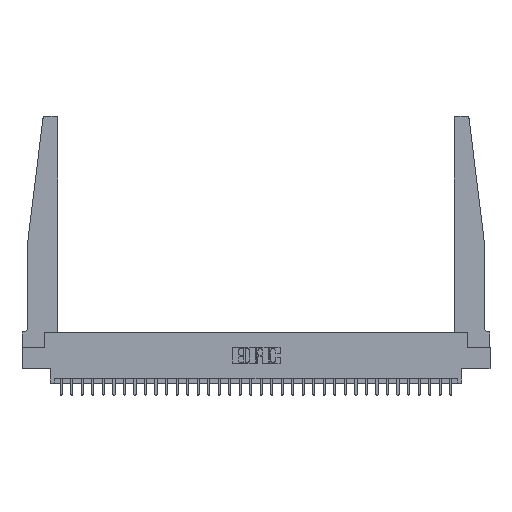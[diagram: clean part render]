
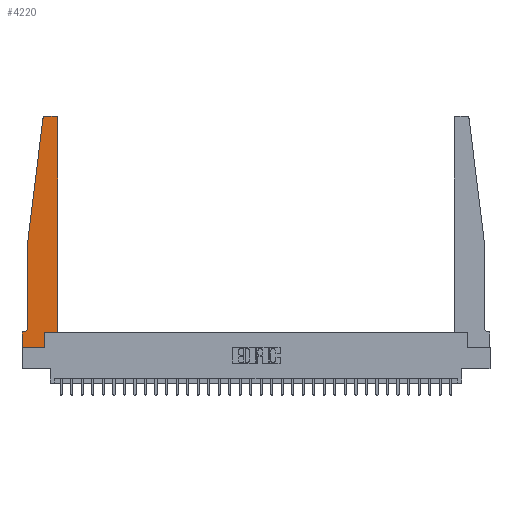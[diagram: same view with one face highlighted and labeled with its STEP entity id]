
A CAD part, top view. The second image highlights one B-rep face of the part: STEP entity #4220.
In plain terms, the highlighted planar face has unit normal (0, 0, 1).
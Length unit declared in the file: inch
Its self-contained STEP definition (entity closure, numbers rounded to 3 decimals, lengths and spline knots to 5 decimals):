
#763 = CARTESIAN_POINT ( 'NONE',  ( 0.065, 1.25, 0.37 ) ) ;
#771 = LINE ( 'NONE', #4137, #20206 ) ;
#1007 = CARTESIAN_POINT ( 'NONE',  ( 0.065, 0.1875, 0.37 ) ) ;
#1200 = CARTESIAN_POINT ( 'NONE',  ( 0., 0., 0.37 ) ) ;
#1254 = ORIENTED_EDGE ( 'NONE', *, *, #18506, .T. ) ;
#1265 = CARTESIAN_POINT ( 'NONE',  ( 0.25, 2.75, 0.37 ) ) ;
#2044 = EDGE_CURVE ( 'NONE', #14643, #9966, #5174, .T. ) ;
#2944 = CIRCLE ( 'NONE', #4883, 0.03 ) ;
#3157 = VERTEX_POINT ( 'NONE', #4139 ) ;
#3623 = DIRECTION ( 'NONE',  ( 1., 0., 0. ) ) ;
#4073 = VERTEX_POINT ( 'NONE', #13093 ) ;
#4137 = CARTESIAN_POINT ( 'NONE',  ( 0.425, 0.18, 0.37 ) ) ;
#4139 = CARTESIAN_POINT ( 'NONE',  ( 0.27653, 2.75, 0.37 ) ) ;
#4220 = ADVANCED_FACE ( 'NONE', ( #11741 ), #6503, .T. ) ;
#4426 = ORIENTED_EDGE ( 'NONE', *, *, #29003, .T. ) ;
#4660 = CIRCLE ( 'NONE', #13501, 0.05 ) ;
#4741 = CARTESIAN_POINT ( 'NONE',  ( 0.065, 1.25, 0.37 ) ) ;
#4878 = EDGE_LOOP ( 'NONE', ( #24129, #21483, #20817, #18148, #17324, #16558, #15035, #14116, #15238, #4426, #1254, #26057 ) ) ;
#4883 = AXIS2_PLACEMENT_3D ( 'NONE', #27953, #14110, #22175 ) ;
#5174 = LINE ( 'NONE', #13880, #23078 ) ;
#6503 = PLANE ( 'NONE',  #27373 ) ;
#6595 = EDGE_CURVE ( 'NONE', #9418, #3157, #24616, .T. ) ;
#7225 = CARTESIAN_POINT ( 'NONE',  ( 0.2605, 0.18, 0.37 ) ) ;
#7365 = CARTESIAN_POINT ( 'NONE',  ( 0., 0.1875, 0.37 ) ) ;
#7398 = VECTOR ( 'NONE', #29221, 39.37008 ) ;
#7646 = CARTESIAN_POINT ( 'NONE',  ( 0.015, 0.2375, 0.37 ) ) ;
#8874 = LINE ( 'NONE', #24558, #7398 ) ;
#9066 = CARTESIAN_POINT ( 'NONE',  ( 0.425, 0.18, 0.37 ) ) ;
#9418 = VERTEX_POINT ( 'NONE', #24285 ) ;
#9519 = DIRECTION ( 'NONE',  ( 0., -1., 0. ) ) ;
#9615 = CARTESIAN_POINT ( 'NONE',  ( 0.395, 2.72, 0.37 ) ) ;
#9966 = VERTEX_POINT ( 'NONE', #7225 ) ;
#10016 = DIRECTION ( 'NONE',  ( -1., 0., 0. ) ) ;
#10546 = DIRECTION ( 'NONE',  ( -1., 0., 0. ) ) ;
#10548 = VECTOR ( 'NONE', #20623, 39.37008 ) ;
#10881 = EDGE_CURVE ( 'NONE', #4073, #11976, #8874, .T. ) ;
#11104 = VERTEX_POINT ( 'NONE', #13737 ) ;
#11255 = DIRECTION ( 'NONE',  ( 1., 0., 0. ) ) ;
#11291 = LINE ( 'NONE', #9066, #10548 ) ;
#11741 = FACE_OUTER_BOUND ( 'NONE', #4878, .T. ) ;
#11976 = VERTEX_POINT ( 'NONE', #763 ) ;
#11994 = DIRECTION ( 'NONE',  ( 1., 0., 0. ) ) ;
#12326 = VECTOR ( 'NONE', #20113, 39.37008 ) ;
#12801 = VECTOR ( 'NONE', #9519, 39.37008 ) ;
#13093 = CARTESIAN_POINT ( 'NONE',  ( 0.24675, 2.72367, 0.37 ) ) ;
#13096 = VERTEX_POINT ( 'NONE', #24035 ) ;
#13266 = EDGE_CURVE ( 'NONE', #11104, #14643, #14215, .T. ) ;
#13501 = AXIS2_PLACEMENT_3D ( 'NONE', #7646, #23896, #10016 ) ;
#13520 = LINE ( 'NONE', #4741, #19624 ) ;
#13659 = EDGE_CURVE ( 'NONE', #22951, #9418, #28666, .T. ) ;
#13737 = CARTESIAN_POINT ( 'NONE',  ( 0., 0., 0.37 ) ) ;
#13880 = CARTESIAN_POINT ( 'NONE',  ( 0.2605, 0.18, 0.37 ) ) ;
#14110 = DIRECTION ( 'NONE',  ( 0., 0., 1. ) ) ;
#14116 = ORIENTED_EDGE ( 'NONE', *, *, #13266, .T. ) ;
#14215 = LINE ( 'NONE', #1200, #20348 ) ;
#14643 = VERTEX_POINT ( 'NONE', #15445 ) ;
#15035 = ORIENTED_EDGE ( 'NONE', *, *, #17964, .T. ) ;
#15238 = ORIENTED_EDGE ( 'NONE', *, *, #2044, .T. ) ;
#15445 = CARTESIAN_POINT ( 'NONE',  ( 0.2605, 0., 0.37 ) ) ;
#15992 = EDGE_CURVE ( 'NONE', #3157, #4073, #2944, .T. ) ;
#16558 = ORIENTED_EDGE ( 'NONE', *, *, #23615, .T. ) ;
#17151 = VECTOR ( 'NONE', #10546, 39.37008 ) ;
#17324 = ORIENTED_EDGE ( 'NONE', *, *, #24159, .T. ) ;
#17949 = EDGE_CURVE ( 'NONE', #11976, #13096, #13520, .T. ) ;
#17964 = EDGE_CURVE ( 'NONE', #25194, #11104, #25092, .T. ) ;
#18148 = ORIENTED_EDGE ( 'NONE', *, *, #17949, .T. ) ;
#18357 = AXIS2_PLACEMENT_3D ( 'NONE', #9615, #25821, #11994 ) ;
#18506 = EDGE_CURVE ( 'NONE', #20076, #22951, #11291, .T. ) ;
#19624 = VECTOR ( 'NONE', #27958, 39.37008 ) ;
#20076 = VERTEX_POINT ( 'NONE', #28711 ) ;
#20113 = DIRECTION ( 'NONE',  ( -1., 0., 0. ) ) ;
#20206 = VECTOR ( 'NONE', #20478, 39.37008 ) ;
#20348 = VECTOR ( 'NONE', #3623, 39.37008 ) ;
#20478 = DIRECTION ( 'NONE',  ( 1., 0., 0. ) ) ;
#20623 = DIRECTION ( 'NONE',  ( 0., 1., 0. ) ) ;
#20817 = ORIENTED_EDGE ( 'NONE', *, *, #10881, .T. ) ;
#20852 = DIRECTION ( 'NONE',  ( 0., 1., 0. ) ) ;
#21483 = ORIENTED_EDGE ( 'NONE', *, *, #15992, .T. ) ;
#22175 = DIRECTION ( 'NONE',  ( 1., 0., 0. ) ) ;
#22798 = CARTESIAN_POINT ( 'NONE',  ( 0., 0.1875, 0.37 ) ) ;
#22951 = VERTEX_POINT ( 'NONE', #24165 ) ;
#23078 = VECTOR ( 'NONE', #20852, 39.37008 ) ;
#23615 = EDGE_CURVE ( 'NONE', #26681, #25194, #29475, .T. ) ;
#23896 = DIRECTION ( 'NONE',  ( 0., 0., -1. ) ) ;
#24035 = CARTESIAN_POINT ( 'NONE',  ( 0.065, 0.2375, 0.37 ) ) ;
#24129 = ORIENTED_EDGE ( 'NONE', *, *, #6595, .T. ) ;
#24159 = EDGE_CURVE ( 'NONE', #13096, #26681, #4660, .T. ) ;
#24165 = CARTESIAN_POINT ( 'NONE',  ( 0.425, 2.72, 0.37 ) ) ;
#24285 = CARTESIAN_POINT ( 'NONE',  ( 0.395, 2.75, 0.37 ) ) ;
#24558 = CARTESIAN_POINT ( 'NONE',  ( 0.065, 1.25, 0.37 ) ) ;
#24616 = LINE ( 'NONE', #1265, #12326 ) ;
#25092 = LINE ( 'NONE', #25729, #12801 ) ;
#25129 = DIRECTION ( 'NONE',  ( 0., 0., 1. ) ) ;
#25194 = VERTEX_POINT ( 'NONE', #7365 ) ;
#25729 = CARTESIAN_POINT ( 'NONE',  ( 0., 0., 0.37 ) ) ;
#25821 = DIRECTION ( 'NONE',  ( 0., 0., 1. ) ) ;
#26057 = ORIENTED_EDGE ( 'NONE', *, *, #13659, .T. ) ;
#26681 = VERTEX_POINT ( 'NONE', #29406 ) ;
#27373 = AXIS2_PLACEMENT_3D ( 'NONE', #22798, #25129, #11255 ) ;
#27953 = CARTESIAN_POINT ( 'NONE',  ( 0.27653, 2.72, 0.37 ) ) ;
#27958 = DIRECTION ( 'NONE',  ( 0., -1., 0. ) ) ;
#28666 = CIRCLE ( 'NONE', #18357, 0.03 ) ;
#28711 = CARTESIAN_POINT ( 'NONE',  ( 0.425, 0.18, 0.37 ) ) ;
#29003 = EDGE_CURVE ( 'NONE', #9966, #20076, #771, .T. ) ;
#29221 = DIRECTION ( 'NONE',  ( -0.122, -0.992, 0. ) ) ;
#29406 = CARTESIAN_POINT ( 'NONE',  ( 0.015, 0.1875, 0.37 ) ) ;
#29475 = LINE ( 'NONE', #1007, #17151 ) ;
